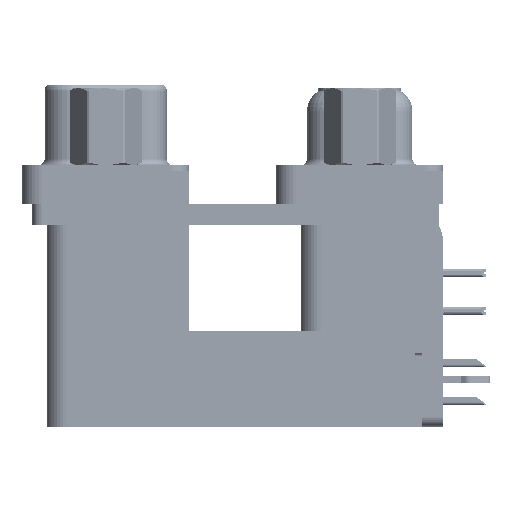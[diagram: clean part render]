
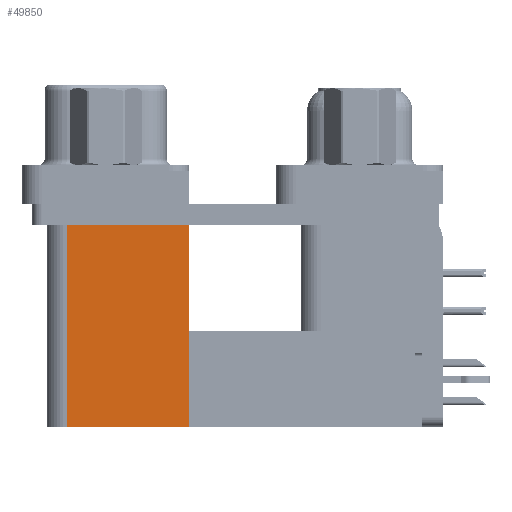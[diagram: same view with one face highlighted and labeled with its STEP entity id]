
A CAD part, left-side view. The second image highlights one B-rep face of the part: STEP entity #49850.
In plain terms, the highlighted planar face has unit normal (-1, 0, 0).
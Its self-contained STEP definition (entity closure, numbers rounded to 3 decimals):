
#350 = VECTOR ( 'NONE', #13852, 1000. ) ;
#480 = EDGE_CURVE ( 'NONE', #14496, #33475, #25612, .T. ) ;
#5867 = EDGE_CURVE ( 'NONE', #33475, #23004, #60866, .T. ) ;
#7720 = PLANE ( 'NONE',  #45064 ) ;
#8926 = EDGE_LOOP ( 'NONE', ( #32889, #14397, #53263, #57047 ) ) ;
#11173 = CARTESIAN_POINT ( 'NONE',  ( 3.7, 12.775, -2.5 ) ) ;
#11214 = EDGE_CURVE ( 'NONE', #49486, #23004, #59666, .T. ) ;
#11595 = CARTESIAN_POINT ( 'NONE',  ( 3.7, 12.775, -19.2 ) ) ;
#13852 = DIRECTION ( 'NONE',  ( 0., 1., 0. ) ) ;
#14397 = ORIENTED_EDGE ( 'NONE', *, *, #5867, .F. ) ;
#14496 = VERTEX_POINT ( 'NONE', #51352 ) ;
#17741 = CARTESIAN_POINT ( 'NONE',  ( 3.7, 12.775, -19.2 ) ) ;
#23004 = VERTEX_POINT ( 'NONE', #32173 ) ;
#25612 = LINE ( 'NONE', #11595, #33620 ) ;
#32173 = CARTESIAN_POINT ( 'NONE',  ( 3.7, 21.975, -2.5 ) ) ;
#32889 = ORIENTED_EDGE ( 'NONE', *, *, #11214, .T. ) ;
#33475 = VERTEX_POINT ( 'NONE', #56737 ) ;
#33620 = VECTOR ( 'NONE', #34355, 1000. ) ;
#34355 = DIRECTION ( 'NONE',  ( 0., 1., 0. ) ) ;
#40817 = DIRECTION ( 'NONE',  ( 0., 0., 1. ) ) ;
#40985 = VECTOR ( 'NONE', #40817, 1000. ) ;
#42587 = CARTESIAN_POINT ( 'NONE',  ( 3.7, 12.775, -19.2 ) ) ;
#45064 = AXIS2_PLACEMENT_3D ( 'NONE', #42587, #56003, #47259 ) ;
#46441 = VECTOR ( 'NONE', #49302, 1000. ) ;
#46868 = CARTESIAN_POINT ( 'NONE',  ( 3.7, 12.775, -2.5 ) ) ;
#47259 = DIRECTION ( 'NONE',  ( 0., 1., 0. ) ) ;
#48082 = EDGE_CURVE ( 'NONE', #14496, #49486, #50475, .T. ) ;
#49302 = DIRECTION ( 'NONE',  ( 0., 0., 1. ) ) ;
#49486 = VERTEX_POINT ( 'NONE', #11173 ) ;
#49850 = ADVANCED_FACE ( 'NONE', ( #50406 ), #7720, .F. ) ;
#50406 = FACE_OUTER_BOUND ( 'NONE', #8926, .T. ) ;
#50475 = LINE ( 'NONE', #17741, #40985 ) ;
#51352 = CARTESIAN_POINT ( 'NONE',  ( 3.7, 12.775, -19.2 ) ) ;
#53263 = ORIENTED_EDGE ( 'NONE', *, *, #480, .F. ) ;
#56003 = DIRECTION ( 'NONE',  ( 1., 0., 0. ) ) ;
#56737 = CARTESIAN_POINT ( 'NONE',  ( 3.7, 21.975, -19.2 ) ) ;
#57047 = ORIENTED_EDGE ( 'NONE', *, *, #48082, .T. ) ;
#57744 = CARTESIAN_POINT ( 'NONE',  ( 3.7, 21.975, -19.2 ) ) ;
#59666 = LINE ( 'NONE', #46868, #350 ) ;
#60866 = LINE ( 'NONE', #57744, #46441 ) ;
